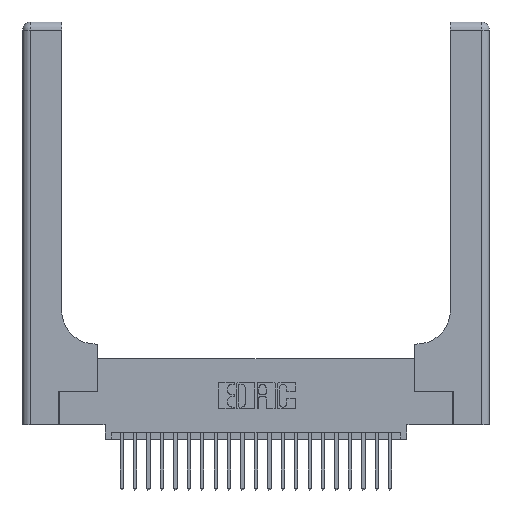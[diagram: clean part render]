
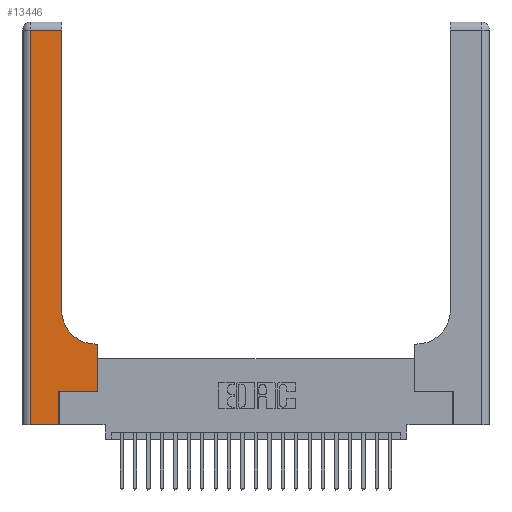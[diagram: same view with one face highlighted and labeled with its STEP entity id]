
A CAD part, top view. The second image highlights one B-rep face of the part: STEP entity #13446.
In plain terms, the highlighted planar face has unit normal (0, 0, 1).
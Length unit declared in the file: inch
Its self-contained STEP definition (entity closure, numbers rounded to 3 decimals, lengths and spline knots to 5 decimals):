
#153 = DIRECTION ( 'NONE',  ( 0., -1., 0. ) ) ;
#297 = EDGE_CURVE ( 'NONE', #3733, #14044, #4476, .T. ) ;
#500 = DIRECTION ( 'NONE',  ( 1., 0., 0. ) ) ;
#559 = VECTOR ( 'NONE', #19463, 39.37008 ) ;
#726 = VECTOR ( 'NONE', #153, 39.37008 ) ;
#1080 = CARTESIAN_POINT ( 'NONE',  ( 0.5585, 0.25, 0.37 ) ) ;
#1464 = EDGE_CURVE ( 'NONE', #15649, #20300, #8258, .T. ) ;
#1571 = VERTEX_POINT ( 'NONE', #4071 ) ;
#1576 = AXIS2_PLACEMENT_3D ( 'NONE', #3264, #11197, #500 ) ;
#1712 = CARTESIAN_POINT ( 'NONE',  ( 0., 3., 0.37 ) ) ;
#1818 = CARTESIAN_POINT ( 'NONE',  ( 0.5585, 0.6, 0.37 ) ) ;
#2114 = EDGE_CURVE ( 'NONE', #17759, #13484, #4961, .T. ) ;
#2340 = DIRECTION ( 'NONE',  ( 0., 1., 0. ) ) ;
#2493 = LINE ( 'NONE', #3416, #726 ) ;
#3264 = CARTESIAN_POINT ( 'NONE',  ( 0.5415, 0.85, 0.37 ) ) ;
#3416 = CARTESIAN_POINT ( 'NONE',  ( 0.06, 3., 0.37 ) ) ;
#3733 = VERTEX_POINT ( 'NONE', #14439 ) ;
#4031 = VERTEX_POINT ( 'NONE', #21740 ) ;
#4071 = CARTESIAN_POINT ( 'NONE',  ( 0.269, 0.25, 0.37 ) ) ;
#4186 = ORIENTED_EDGE ( 'NONE', *, *, #297, .T. ) ;
#4373 = FACE_OUTER_BOUND ( 'NONE', #20034, .T. ) ;
#4408 = CIRCLE ( 'NONE', #1576, 0.25 ) ;
#4476 = LINE ( 'NONE', #9674, #24160 ) ;
#4855 = LINE ( 'NONE', #1080, #15216 ) ;
#4961 = LINE ( 'NONE', #12318, #21004 ) ;
#5200 = LINE ( 'NONE', #20275, #23691 ) ;
#5233 = ORIENTED_EDGE ( 'NONE', *, *, #10250, .T. ) ;
#5541 = CARTESIAN_POINT ( 'NONE',  ( 0., 2.94, 0.37 ) ) ;
#5651 = EDGE_CURVE ( 'NONE', #1571, #4031, #5200, .T. ) ;
#7622 = CARTESIAN_POINT ( 'NONE',  ( 0.2915, 0.85, 0.37 ) ) ;
#7692 = EDGE_CURVE ( 'NONE', #14044, #1571, #14319, .T. ) ;
#7745 = DIRECTION ( 'NONE',  ( -1., 0., 0. ) ) ;
#8258 = LINE ( 'NONE', #5541, #24370 ) ;
#8565 = ORIENTED_EDGE ( 'NONE', *, *, #18401, .T. ) ;
#9292 = VECTOR ( 'NONE', #2340, 39.37008 ) ;
#9674 = CARTESIAN_POINT ( 'NONE',  ( 0., 0., 0.37 ) ) ;
#9812 = CARTESIAN_POINT ( 'NONE',  ( 0.269, 0., 0.37 ) ) ;
#9852 = ORIENTED_EDGE ( 'NONE', *, *, #7692, .T. ) ;
#10230 = EDGE_CURVE ( 'NONE', #13484, #11511, #4408, .T. ) ;
#10250 = EDGE_CURVE ( 'NONE', #11511, #15649, #14488, .T. ) ;
#11197 = DIRECTION ( 'NONE',  ( 0., 0., -1. ) ) ;
#11511 = VERTEX_POINT ( 'NONE', #7622 ) ;
#12006 = CARTESIAN_POINT ( 'NONE',  ( 0.06, 2.94, 0.37 ) ) ;
#12053 = CARTESIAN_POINT ( 'NONE',  ( 0.269, 0., 0.37 ) ) ;
#12318 = CARTESIAN_POINT ( 'NONE',  ( 0.2915, 0.6, 0.37 ) ) ;
#12565 = CARTESIAN_POINT ( 'NONE',  ( 0.5415, 0.6, 0.37 ) ) ;
#12879 = DIRECTION ( 'NONE',  ( 1., 0., 0. ) ) ;
#13150 = DIRECTION ( 'NONE',  ( 0., 0., -1. ) ) ;
#13446 = ADVANCED_FACE ( 'NONE', ( #4373 ), #16967, .F. ) ;
#13484 = VERTEX_POINT ( 'NONE', #12565 ) ;
#13490 = DIRECTION ( 'NONE',  ( 1., 0., 0. ) ) ;
#14044 = VERTEX_POINT ( 'NONE', #12053 ) ;
#14319 = LINE ( 'NONE', #9812, #9292 ) ;
#14439 = CARTESIAN_POINT ( 'NONE',  ( 0.06, 0., 0.37 ) ) ;
#14488 = LINE ( 'NONE', #17459, #559 ) ;
#15216 = VECTOR ( 'NONE', #18177, 39.37008 ) ;
#15645 = ORIENTED_EDGE ( 'NONE', *, *, #18666, .T. ) ;
#15649 = VERTEX_POINT ( 'NONE', #22692 ) ;
#15969 = ORIENTED_EDGE ( 'NONE', *, *, #2114, .T. ) ;
#16967 = PLANE ( 'NONE',  #18957 ) ;
#17459 = CARTESIAN_POINT ( 'NONE',  ( 0.2915, 3., 0.37 ) ) ;
#17759 = VERTEX_POINT ( 'NONE', #1818 ) ;
#18177 = DIRECTION ( 'NONE',  ( 0., 1., 0. ) ) ;
#18401 = EDGE_CURVE ( 'NONE', #20300, #3733, #2493, .T. ) ;
#18666 = EDGE_CURVE ( 'NONE', #4031, #17759, #4855, .T. ) ;
#18957 = AXIS2_PLACEMENT_3D ( 'NONE', #1712, #13150, #18983 ) ;
#18983 = DIRECTION ( 'NONE',  ( -1., 0., 0. ) ) ;
#19463 = DIRECTION ( 'NONE',  ( 0., 1., 0. ) ) ;
#19692 = ORIENTED_EDGE ( 'NONE', *, *, #1464, .T. ) ;
#20034 = EDGE_LOOP ( 'NONE', ( #5233, #19692, #8565, #4186, #9852, #20266, #15645, #15969, #24625 ) ) ;
#20266 = ORIENTED_EDGE ( 'NONE', *, *, #5651, .T. ) ;
#20275 = CARTESIAN_POINT ( 'NONE',  ( 0.269, 0.25, 0.37 ) ) ;
#20300 = VERTEX_POINT ( 'NONE', #12006 ) ;
#21004 = VECTOR ( 'NONE', #7745, 39.37008 ) ;
#21740 = CARTESIAN_POINT ( 'NONE',  ( 0.5585, 0.25, 0.37 ) ) ;
#22692 = CARTESIAN_POINT ( 'NONE',  ( 0.2915, 2.94, 0.37 ) ) ;
#22710 = DIRECTION ( 'NONE',  ( -1., 0., 0. ) ) ;
#23691 = VECTOR ( 'NONE', #12879, 39.37008 ) ;
#24160 = VECTOR ( 'NONE', #13490, 39.37008 ) ;
#24370 = VECTOR ( 'NONE', #22710, 39.37008 ) ;
#24625 = ORIENTED_EDGE ( 'NONE', *, *, #10230, .T. ) ;
